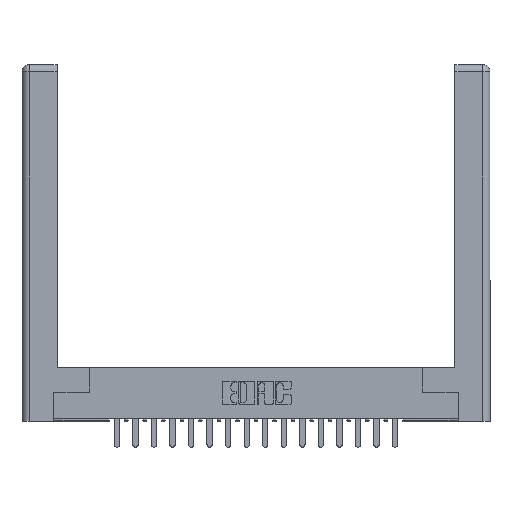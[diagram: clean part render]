
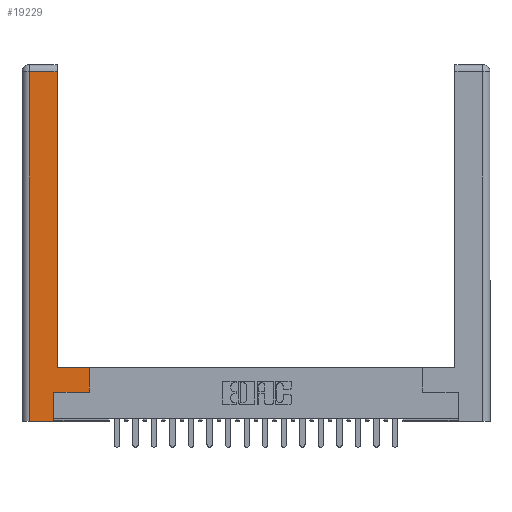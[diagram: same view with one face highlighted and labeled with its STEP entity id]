
A CAD part, top view. The second image highlights one B-rep face of the part: STEP entity #19229.
In plain terms, the highlighted planar face has unit normal (0, 0, 1).
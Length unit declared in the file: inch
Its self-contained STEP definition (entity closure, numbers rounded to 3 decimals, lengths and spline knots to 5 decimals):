
#270 = VECTOR ( 'NONE', #16818, 39.37008 ) ;
#668 = VERTEX_POINT ( 'NONE', #15612 ) ;
#678 = CARTESIAN_POINT ( 'NONE',  ( 0.295, 2.94, 0. ) ) ;
#987 = DIRECTION ( 'NONE',  ( 1., 0., 0. ) ) ;
#1150 = CARTESIAN_POINT ( 'NONE',  ( 0.265, 0., 0. ) ) ;
#1532 = ORIENTED_EDGE ( 'NONE', *, *, #16017, .T. ) ;
#2244 = EDGE_LOOP ( 'NONE', ( #20327, #17167, #3702, #1532, #8537, #20274, #3813, #22252 ) ) ;
#2295 = EDGE_CURVE ( 'NONE', #14910, #5941, #17046, .T. ) ;
#2300 = CARTESIAN_POINT ( 'NONE',  ( 0.295, 0.45, 0. ) ) ;
#2379 = DIRECTION ( 'NONE',  ( -1., 0., 0. ) ) ;
#2459 = VECTOR ( 'NONE', #19907, 39.37008 ) ;
#3042 = VERTEX_POINT ( 'NONE', #18132 ) ;
#3702 = ORIENTED_EDGE ( 'NONE', *, *, #6201, .T. ) ;
#3813 = ORIENTED_EDGE ( 'NONE', *, *, #21880, .T. ) ;
#4322 = CARTESIAN_POINT ( 'NONE',  ( 0.265, 0., 0. ) ) ;
#5487 = LINE ( 'NONE', #2300, #2459 ) ;
#5941 = VERTEX_POINT ( 'NONE', #15604 ) ;
#6201 = EDGE_CURVE ( 'NONE', #5941, #668, #18082, .T. ) ;
#6688 = DIRECTION ( 'NONE',  ( 0., 1., 0. ) ) ;
#7213 = VERTEX_POINT ( 'NONE', #19088 ) ;
#7480 = DIRECTION ( 'NONE',  ( 0., 1., 0. ) ) ;
#7839 = CARTESIAN_POINT ( 'NONE',  ( 0.0615, 0., 0. ) ) ;
#7917 = LINE ( 'NONE', #18426, #18551 ) ;
#8019 = EDGE_CURVE ( 'NONE', #14236, #12078, #12139, .T. ) ;
#8376 = EDGE_CURVE ( 'NONE', #7213, #14910, #7917, .T. ) ;
#8528 = LINE ( 'NONE', #20613, #10508 ) ;
#8537 = ORIENTED_EDGE ( 'NONE', *, *, #18031, .T. ) ;
#8744 = DIRECTION ( 'NONE',  ( 1., 0., 0. ) ) ;
#10213 = VECTOR ( 'NONE', #8744, 39.37008 ) ;
#10366 = EDGE_CURVE ( 'NONE', #3042, #7213, #5487, .T. ) ;
#10508 = VECTOR ( 'NONE', #17715, 39.37008 ) ;
#10841 = VECTOR ( 'NONE', #987, 39.37008 ) ;
#11326 = CARTESIAN_POINT ( 'NONE',  ( 0., 0., 0. ) ) ;
#12077 = CARTESIAN_POINT ( 'NONE',  ( 0.265, 0.245, 0. ) ) ;
#12078 = VERTEX_POINT ( 'NONE', #21919 ) ;
#12139 = LINE ( 'NONE', #17602, #10213 ) ;
#13318 = VERTEX_POINT ( 'NONE', #4322 ) ;
#14236 = VERTEX_POINT ( 'NONE', #22206 ) ;
#14729 = CARTESIAN_POINT ( 'NONE',  ( 0.0615, 2.94, 0. ) ) ;
#14910 = VERTEX_POINT ( 'NONE', #678 ) ;
#15163 = DIRECTION ( 'NONE',  ( 0., 0., -1. ) ) ;
#15429 = VECTOR ( 'NONE', #6688, 39.37008 ) ;
#15600 = LINE ( 'NONE', #1150, #10841 ) ;
#15604 = CARTESIAN_POINT ( 'NONE',  ( 0.0615, 2.94, 0. ) ) ;
#15612 = CARTESIAN_POINT ( 'NONE',  ( 0.0615, 0., 0. ) ) ;
#16017 = EDGE_CURVE ( 'NONE', #668, #13318, #15600, .T. ) ;
#16818 = DIRECTION ( 'NONE',  ( 0., -1., 0. ) ) ;
#17046 = LINE ( 'NONE', #14729, #20362 ) ;
#17167 = ORIENTED_EDGE ( 'NONE', *, *, #2295, .T. ) ;
#17602 = CARTESIAN_POINT ( 'NONE',  ( 0.565, 0.245, 0. ) ) ;
#17715 = DIRECTION ( 'NONE',  ( 0., 1., 0. ) ) ;
#18031 = EDGE_CURVE ( 'NONE', #13318, #14236, #19320, .T. ) ;
#18082 = LINE ( 'NONE', #7839, #270 ) ;
#18132 = CARTESIAN_POINT ( 'NONE',  ( 0.565, 0.45, 0. ) ) ;
#18426 = CARTESIAN_POINT ( 'NONE',  ( 0.295, 3., 0. ) ) ;
#18551 = VECTOR ( 'NONE', #7480, 39.37008 ) ;
#18946 = AXIS2_PLACEMENT_3D ( 'NONE', #11326, #15163, #2379 ) ;
#19088 = CARTESIAN_POINT ( 'NONE',  ( 0.295, 0.45, 0. ) ) ;
#19229 = ADVANCED_FACE ( 'NONE', ( #19564 ), #20130, .F. ) ;
#19320 = LINE ( 'NONE', #12077, #15429 ) ;
#19564 = FACE_OUTER_BOUND ( 'NONE', #2244, .T. ) ;
#19907 = DIRECTION ( 'NONE',  ( -1., 0., 0. ) ) ;
#20083 = DIRECTION ( 'NONE',  ( -1., 0., 0. ) ) ;
#20130 = PLANE ( 'NONE',  #18946 ) ;
#20274 = ORIENTED_EDGE ( 'NONE', *, *, #8019, .T. ) ;
#20327 = ORIENTED_EDGE ( 'NONE', *, *, #8376, .T. ) ;
#20362 = VECTOR ( 'NONE', #20083, 39.37008 ) ;
#20613 = CARTESIAN_POINT ( 'NONE',  ( 0.565, 0.45, 0. ) ) ;
#21880 = EDGE_CURVE ( 'NONE', #12078, #3042, #8528, .T. ) ;
#21919 = CARTESIAN_POINT ( 'NONE',  ( 0.565, 0.245, 0. ) ) ;
#22206 = CARTESIAN_POINT ( 'NONE',  ( 0.265, 0.245, 0. ) ) ;
#22252 = ORIENTED_EDGE ( 'NONE', *, *, #10366, .T. ) ;
